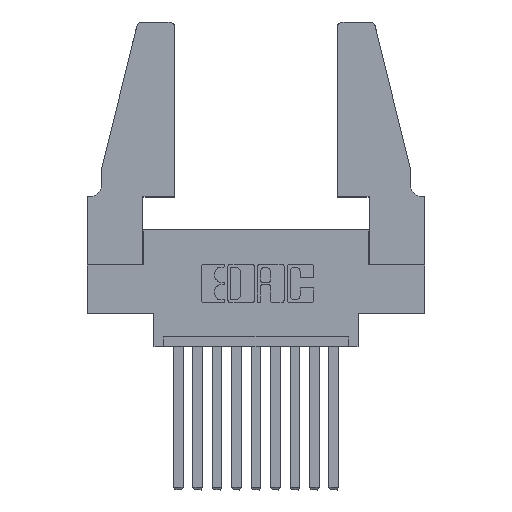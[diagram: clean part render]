
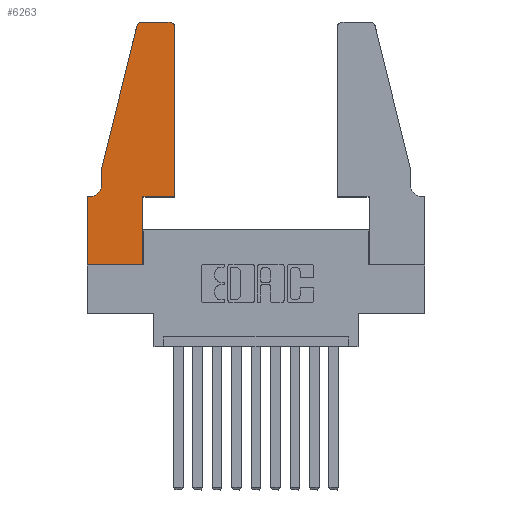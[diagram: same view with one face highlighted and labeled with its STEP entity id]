
A CAD part, top view. The second image highlights one B-rep face of the part: STEP entity #6263.
In plain terms, the highlighted planar face has unit normal (0, 0, 1).
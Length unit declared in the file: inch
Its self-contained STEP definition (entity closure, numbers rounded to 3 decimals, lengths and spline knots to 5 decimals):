
#173 = AXIS2_PLACEMENT_3D ( 'NONE', #1134, #2150, #4125 ) ;
#443 = EDGE_CURVE ( 'NONE', #2146, #7192, #11273, .T. ) ;
#476 = DIRECTION ( 'NONE',  ( 1., 0., 0. ) ) ;
#573 = CARTESIAN_POINT ( 'NONE',  ( 0.2865, 0.35, 0.37 ) ) ;
#610 = VERTEX_POINT ( 'NONE', #4399 ) ;
#854 = VECTOR ( 'NONE', #2172, 39.37008 ) ;
#948 = CARTESIAN_POINT ( 'NONE',  ( 0.4505, 0.35, 0.37 ) ) ;
#1105 = DIRECTION ( 'NONE',  ( 0., 1., 0. ) ) ;
#1134 = CARTESIAN_POINT ( 'NONE',  ( 0., 0.35, 0.37 ) ) ;
#1677 = ORIENTED_EDGE ( 'NONE', *, *, #8402, .T. ) ;
#1908 = ORIENTED_EDGE ( 'NONE', *, *, #10364, .T. ) ;
#1925 = ORIENTED_EDGE ( 'NONE', *, *, #2926, .T. ) ;
#2146 = VERTEX_POINT ( 'NONE', #7577 ) ;
#2150 = DIRECTION ( 'NONE',  ( 0., 0., 1. ) ) ;
#2151 = LINE ( 'NONE', #11780, #13240 ) ;
#2172 = DIRECTION ( 'NONE',  ( -0.239, -0.971, 0. ) ) ;
#2261 = CARTESIAN_POINT ( 'NONE',  ( 0.0755, 0.5, 0.37 ) ) ;
#2835 = LINE ( 'NONE', #10924, #5076 ) ;
#2851 = DIRECTION ( 'NONE',  ( 0., -1., 0. ) ) ;
#2926 = EDGE_CURVE ( 'NONE', #4498, #4587, #3202, .T. ) ;
#2963 = ORIENTED_EDGE ( 'NONE', *, *, #5376, .T. ) ;
#2995 = ORIENTED_EDGE ( 'NONE', *, *, #443, .T. ) ;
#3198 = DIRECTION ( 'NONE',  ( 0., 0., 1. ) ) ;
#3202 = LINE ( 'NONE', #11261, #7709 ) ;
#3372 = CARTESIAN_POINT ( 'NONE',  ( 0.0755, 0.42, 0.37 ) ) ;
#3472 = LINE ( 'NONE', #10173, #10378 ) ;
#3574 = ORIENTED_EDGE ( 'NONE', *, *, #13207, .T. ) ;
#3647 = ORIENTED_EDGE ( 'NONE', *, *, #4796, .T. ) ;
#4096 = FACE_OUTER_BOUND ( 'NONE', #9026, .T. ) ;
#4125 = DIRECTION ( 'NONE',  ( 1., 0., 0. ) ) ;
#4128 = EDGE_CURVE ( 'NONE', #610, #11726, #11213, .T. ) ;
#4150 = CARTESIAN_POINT ( 'NONE',  ( 0.0055, 0.42, 0.37 ) ) ;
#4389 = ORIENTED_EDGE ( 'NONE', *, *, #7224, .T. ) ;
#4394 = VERTEX_POINT ( 'NONE', #12046 ) ;
#4399 = CARTESIAN_POINT ( 'NONE',  ( 0.284, 1.25, 0.37 ) ) ;
#4498 = VERTEX_POINT ( 'NONE', #10035 ) ;
#4540 = CARTESIAN_POINT ( 'NONE',  ( 0.4205, 1.22, 0.37 ) ) ;
#4548 = DIRECTION ( 'NONE',  ( 0., 1., 0. ) ) ;
#4587 = VERTEX_POINT ( 'NONE', #6975 ) ;
#4589 = LINE ( 'NONE', #2261, #854 ) ;
#4633 = LINE ( 'NONE', #573, #9742 ) ;
#4796 = EDGE_CURVE ( 'NONE', #4587, #11387, #4633, .T. ) ;
#5064 = DIRECTION ( 'NONE',  ( 0., 0., -1. ) ) ;
#5076 = VECTOR ( 'NONE', #10134, 39.37008 ) ;
#5215 = CARTESIAN_POINT ( 'NONE',  ( 0.4505, 0.35, 0.37 ) ) ;
#5376 = EDGE_CURVE ( 'NONE', #4394, #7525, #7162, .T. ) ;
#5416 = ORIENTED_EDGE ( 'NONE', *, *, #4128, .T. ) ;
#5569 = EDGE_CURVE ( 'NONE', #7525, #4498, #3472, .T. ) ;
#5846 = VECTOR ( 'NONE', #1105, 39.37008 ) ;
#6115 = CARTESIAN_POINT ( 'NONE',  ( 0.0755, 0.5, 0.37 ) ) ;
#6156 = DIRECTION ( 'NONE',  ( -1., 0., 0. ) ) ;
#6192 = VECTOR ( 'NONE', #12260, 39.37008 ) ;
#6263 = ADVANCED_FACE ( 'NONE', ( #4096 ), #10269, .T. ) ;
#6488 = CIRCLE ( 'NONE', #12801, 0.07 ) ;
#6533 = VECTOR ( 'NONE', #7540, 39.37008 ) ;
#6555 = DIRECTION ( 'NONE',  ( 0., 0., 1. ) ) ;
#6975 = CARTESIAN_POINT ( 'NONE',  ( 0.2865, 0., 0.37 ) ) ;
#7030 = AXIS2_PLACEMENT_3D ( 'NONE', #9342, #3198, #10466 ) ;
#7141 = DIRECTION ( 'NONE',  ( 1., 0., 0. ) ) ;
#7162 = LINE ( 'NONE', #13073, #6533 ) ;
#7163 = DIRECTION ( 'NONE',  ( 0., -1., 0. ) ) ;
#7192 = VERTEX_POINT ( 'NONE', #12285 ) ;
#7224 = EDGE_CURVE ( 'NONE', #7911, #4394, #6488, .T. ) ;
#7525 = VERTEX_POINT ( 'NONE', #11825 ) ;
#7540 = DIRECTION ( 'NONE',  ( -1., 0., 0. ) ) ;
#7577 = CARTESIAN_POINT ( 'NONE',  ( 0.4505, 0.35, 0.37 ) ) ;
#7709 = VECTOR ( 'NONE', #7141, 39.37008 ) ;
#7911 = VERTEX_POINT ( 'NONE', #3372 ) ;
#7997 = ORIENTED_EDGE ( 'NONE', *, *, #5569, .T. ) ;
#8187 = EDGE_CURVE ( 'NONE', #9597, #610, #2835, .T. ) ;
#8402 = EDGE_CURVE ( 'NONE', #11726, #9264, #4589, .T. ) ;
#8901 = LINE ( 'NONE', #948, #6192 ) ;
#9026 = EDGE_LOOP ( 'NONE', ( #10545, #5416, #1677, #3574, #4389, #2963, #7997, #1925, #3647, #12828, #2995, #1908 ) ) ;
#9264 = VERTEX_POINT ( 'NONE', #6115 ) ;
#9342 = CARTESIAN_POINT ( 'NONE',  ( 0.284, 1.22, 0.37 ) ) ;
#9487 = CIRCLE ( 'NONE', #11349, 0.03 ) ;
#9597 = VERTEX_POINT ( 'NONE', #12917 ) ;
#9742 = VECTOR ( 'NONE', #4548, 39.37008 ) ;
#10035 = CARTESIAN_POINT ( 'NONE',  ( 0., 0., 0.37 ) ) ;
#10134 = DIRECTION ( 'NONE',  ( -1., 0., 0. ) ) ;
#10173 = CARTESIAN_POINT ( 'NONE',  ( 0., 0., 0.37 ) ) ;
#10243 = CARTESIAN_POINT ( 'NONE',  ( 0.2865, 0.35, 0.37 ) ) ;
#10269 = PLANE ( 'NONE',  #173 ) ;
#10364 = EDGE_CURVE ( 'NONE', #7192, #9597, #9487, .T. ) ;
#10378 = VECTOR ( 'NONE', #7163, 39.37008 ) ;
#10466 = DIRECTION ( 'NONE',  ( 1., 0., 0. ) ) ;
#10545 = ORIENTED_EDGE ( 'NONE', *, *, #8187, .T. ) ;
#10924 = CARTESIAN_POINT ( 'NONE',  ( 0.2605, 1.25, 0.37 ) ) ;
#11213 = CIRCLE ( 'NONE', #7030, 0.03 ) ;
#11261 = CARTESIAN_POINT ( 'NONE',  ( 0., 0., 0.37 ) ) ;
#11273 = LINE ( 'NONE', #5215, #5846 ) ;
#11349 = AXIS2_PLACEMENT_3D ( 'NONE', #4540, #6555, #476 ) ;
#11387 = VERTEX_POINT ( 'NONE', #10243 ) ;
#11550 = CARTESIAN_POINT ( 'NONE',  ( 0.25487, 1.22718, 0.37 ) ) ;
#11726 = VERTEX_POINT ( 'NONE', #11550 ) ;
#11780 = CARTESIAN_POINT ( 'NONE',  ( 0.0755, 0.5, 0.37 ) ) ;
#11825 = CARTESIAN_POINT ( 'NONE',  ( 0., 0.35, 0.37 ) ) ;
#12046 = CARTESIAN_POINT ( 'NONE',  ( 0.0055, 0.35, 0.37 ) ) ;
#12260 = DIRECTION ( 'NONE',  ( 1., 0., 0. ) ) ;
#12285 = CARTESIAN_POINT ( 'NONE',  ( 0.4505, 1.22, 0.37 ) ) ;
#12801 = AXIS2_PLACEMENT_3D ( 'NONE', #4150, #5064, #6156 ) ;
#12828 = ORIENTED_EDGE ( 'NONE', *, *, #13067, .T. ) ;
#12917 = CARTESIAN_POINT ( 'NONE',  ( 0.4205, 1.25, 0.37 ) ) ;
#13067 = EDGE_CURVE ( 'NONE', #11387, #2146, #8901, .T. ) ;
#13073 = CARTESIAN_POINT ( 'NONE',  ( 0.0755, 0.35, 0.37 ) ) ;
#13207 = EDGE_CURVE ( 'NONE', #9264, #7911, #2151, .T. ) ;
#13240 = VECTOR ( 'NONE', #2851, 39.37008 ) ;
